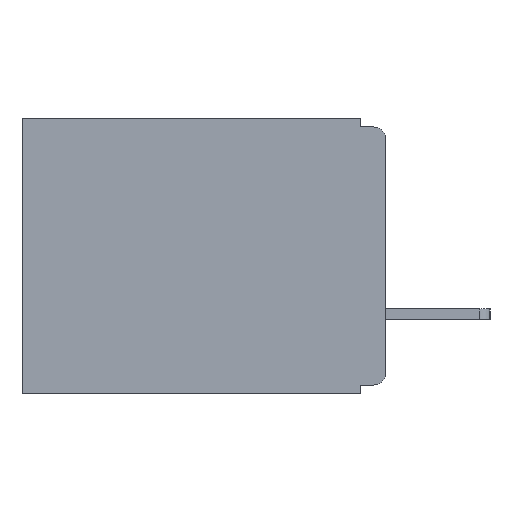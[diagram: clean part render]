
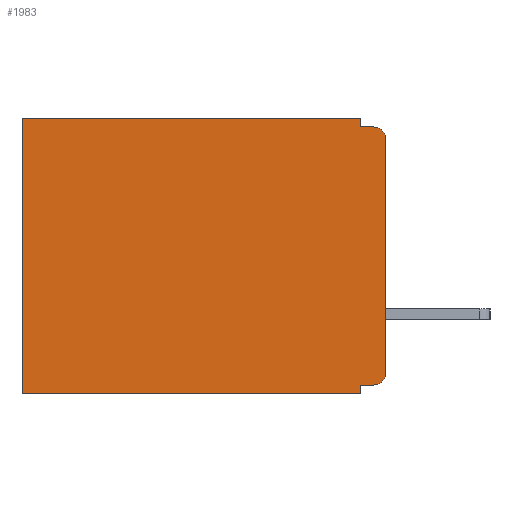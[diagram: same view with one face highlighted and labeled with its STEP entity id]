
A CAD part, left-side view. The second image highlights one B-rep face of the part: STEP entity #1983.
In plain terms, the highlighted planar face has unit normal (-1, 0, 0).
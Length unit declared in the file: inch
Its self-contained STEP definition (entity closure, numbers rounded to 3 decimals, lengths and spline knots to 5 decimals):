
#182 = VERTEX_POINT ( 'NONE', #14871 ) ;
#378 = LINE ( 'NONE', #2279, #7008 ) ;
#653 = AXIS2_PLACEMENT_3D ( 'NONE', #2393, #11573, #3754 ) ;
#817 = EDGE_CURVE ( 'NONE', #12353, #8334, #12691, .T. ) ;
#822 = DIRECTION ( 'NONE',  ( 0., -1., 0. ) ) ;
#845 = VERTEX_POINT ( 'NONE', #3718 ) ;
#933 = CARTESIAN_POINT ( 'NONE',  ( 0.3, 0., -0.025 ) ) ;
#1516 = ORIENTED_EDGE ( 'NONE', *, *, #6280, .F. ) ;
#1528 = LINE ( 'NONE', #14844, #14966 ) ;
#1748 = CARTESIAN_POINT ( 'NONE',  ( 0.3, 0.437, -0.33 ) ) ;
#1969 = CIRCLE ( 'NONE', #2285, 0.015 ) ;
#1983 = ADVANCED_FACE ( 'NONE', ( #3112 ), #8606, .F. ) ;
#2279 = CARTESIAN_POINT ( 'NONE',  ( 0.3, 0.031, 0. ) ) ;
#2285 = AXIS2_PLACEMENT_3D ( 'NONE', #12939, #8139, #10562 ) ;
#2393 = CARTESIAN_POINT ( 'NONE',  ( 0.3, 0.015, -0.025 ) ) ;
#2403 = EDGE_CURVE ( 'NONE', #4834, #3595, #3492, .T. ) ;
#2644 = LINE ( 'NONE', #16457, #8796 ) ;
#3009 = CARTESIAN_POINT ( 'NONE',  ( 0.3, 0., -0.33 ) ) ;
#3031 = ORIENTED_EDGE ( 'NONE', *, *, #8426, .F. ) ;
#3100 = CARTESIAN_POINT ( 'NONE',  ( 0.3, 0.437, -0.33 ) ) ;
#3112 = FACE_OUTER_BOUND ( 'NONE', #10699, .T. ) ;
#3492 = LINE ( 'NONE', #3009, #6972 ) ;
#3595 = VERTEX_POINT ( 'NONE', #4361 ) ;
#3718 = CARTESIAN_POINT ( 'NONE',  ( 0.3, 0.015, -0.01 ) ) ;
#3754 = DIRECTION ( 'NONE',  ( 0., 0., -1. ) ) ;
#4144 = EDGE_CURVE ( 'NONE', #182, #13676, #5508, .T. ) ;
#4159 = EDGE_CURVE ( 'NONE', #16433, #12353, #1528, .T. ) ;
#4361 = CARTESIAN_POINT ( 'NONE',  ( 0.3, 0., -0.305 ) ) ;
#4728 = EDGE_CURVE ( 'NONE', #182, #3595, #1969, .T. ) ;
#4796 = DIRECTION ( 'NONE',  ( 0., 0., -1. ) ) ;
#4834 = VERTEX_POINT ( 'NONE', #933 ) ;
#5267 = ORIENTED_EDGE ( 'NONE', *, *, #4728, .T. ) ;
#5384 = DIRECTION ( 'NONE',  ( 0., 1., 0. ) ) ;
#5508 = LINE ( 'NONE', #13820, #15363 ) ;
#5766 = VECTOR ( 'NONE', #822, 39.37008 ) ;
#6204 = DIRECTION ( 'NONE',  ( 0., 1., 0. ) ) ;
#6236 = CARTESIAN_POINT ( 'NONE',  ( 0.3, 0., -0.33 ) ) ;
#6280 = EDGE_CURVE ( 'NONE', #8551, #8334, #13569, .T. ) ;
#6718 = CARTESIAN_POINT ( 'NONE',  ( 0.3, 0.437, 0. ) ) ;
#6754 = AXIS2_PLACEMENT_3D ( 'NONE', #10287, #8428, #8103 ) ;
#6891 = ORIENTED_EDGE ( 'NONE', *, *, #8950, .F. ) ;
#6972 = VECTOR ( 'NONE', #4796, 39.37008 ) ;
#7008 = VECTOR ( 'NONE', #14439, 39.37008 ) ;
#7086 = VECTOR ( 'NONE', #12249, 39.37008 ) ;
#7297 = ORIENTED_EDGE ( 'NONE', *, *, #2403, .F. ) ;
#7514 = DIRECTION ( 'NONE',  ( 0., 0., -1. ) ) ;
#7893 = ORIENTED_EDGE ( 'NONE', *, *, #4144, .F. ) ;
#8103 = DIRECTION ( 'NONE',  ( 0., 0., -1. ) ) ;
#8138 = ORIENTED_EDGE ( 'NONE', *, *, #12802, .T. ) ;
#8139 = DIRECTION ( 'NONE',  ( -1., 0., 0. ) ) ;
#8255 = CARTESIAN_POINT ( 'NONE',  ( 0.3, 0.031, -0.32 ) ) ;
#8334 = VERTEX_POINT ( 'NONE', #3100 ) ;
#8426 = EDGE_CURVE ( 'NONE', #16433, #10894, #378, .T. ) ;
#8428 = DIRECTION ( 'NONE',  ( 1., 0., 0. ) ) ;
#8459 = CARTESIAN_POINT ( 'NONE',  ( 0.3, 0.031, -0.01 ) ) ;
#8551 = VERTEX_POINT ( 'NONE', #16777 ) ;
#8606 = PLANE ( 'NONE',  #6754 ) ;
#8796 = VECTOR ( 'NONE', #7514, 39.37008 ) ;
#8950 = EDGE_CURVE ( 'NONE', #10894, #845, #12269, .T. ) ;
#10287 = CARTESIAN_POINT ( 'NONE',  ( 0.3, 0., -0.33 ) ) ;
#10409 = CARTESIAN_POINT ( 'NONE',  ( 0.3, 0.031, 0. ) ) ;
#10562 = DIRECTION ( 'NONE',  ( 0., 0., -1. ) ) ;
#10699 = EDGE_LOOP ( 'NONE', ( #7297, #8138, #6891, #3031, #15350, #12786, #1516, #16761, #7893, #5267 ) ) ;
#10894 = VERTEX_POINT ( 'NONE', #8459 ) ;
#11042 = EDGE_CURVE ( 'NONE', #13676, #8551, #2644, .T. ) ;
#11573 = DIRECTION ( 'NONE',  ( -1., 0., 0. ) ) ;
#12249 = DIRECTION ( 'NONE',  ( 0., 1., 0. ) ) ;
#12269 = LINE ( 'NONE', #12874, #5766 ) ;
#12353 = VERTEX_POINT ( 'NONE', #6718 ) ;
#12691 = LINE ( 'NONE', #1748, #15679 ) ;
#12786 = ORIENTED_EDGE ( 'NONE', *, *, #817, .T. ) ;
#12802 = EDGE_CURVE ( 'NONE', #4834, #845, #12967, .T. ) ;
#12874 = CARTESIAN_POINT ( 'NONE',  ( 0.3, 0., -0.01 ) ) ;
#12939 = CARTESIAN_POINT ( 'NONE',  ( 0.3, 0.015, -0.305 ) ) ;
#12967 = CIRCLE ( 'NONE', #653, 0.015 ) ;
#13569 = LINE ( 'NONE', #6236, #7086 ) ;
#13676 = VERTEX_POINT ( 'NONE', #8255 ) ;
#13820 = CARTESIAN_POINT ( 'NONE',  ( 0.3, 0., -0.32 ) ) ;
#14439 = DIRECTION ( 'NONE',  ( 0., 0., -1. ) ) ;
#14844 = CARTESIAN_POINT ( 'NONE',  ( 0.3, 0., 0. ) ) ;
#14871 = CARTESIAN_POINT ( 'NONE',  ( 0.3, 0.015, -0.32 ) ) ;
#14966 = VECTOR ( 'NONE', #5384, 39.37008 ) ;
#14998 = DIRECTION ( 'NONE',  ( 0., 0., -1. ) ) ;
#15350 = ORIENTED_EDGE ( 'NONE', *, *, #4159, .T. ) ;
#15363 = VECTOR ( 'NONE', #6204, 39.37008 ) ;
#15679 = VECTOR ( 'NONE', #14998, 39.37008 ) ;
#16433 = VERTEX_POINT ( 'NONE', #10409 ) ;
#16457 = CARTESIAN_POINT ( 'NONE',  ( 0.3, 0.031, -0.33 ) ) ;
#16761 = ORIENTED_EDGE ( 'NONE', *, *, #11042, .F. ) ;
#16777 = CARTESIAN_POINT ( 'NONE',  ( 0.3, 0.031, -0.33 ) ) ;
